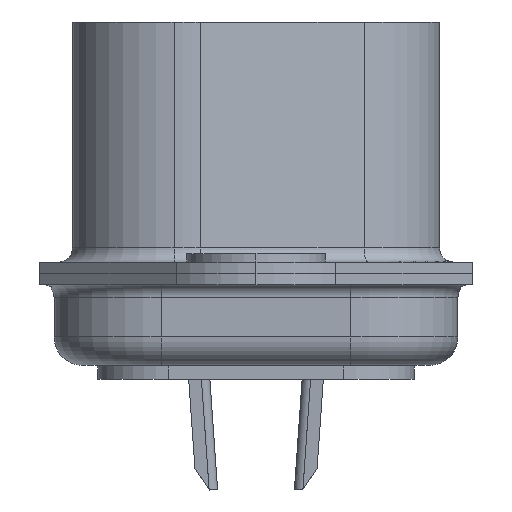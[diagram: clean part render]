
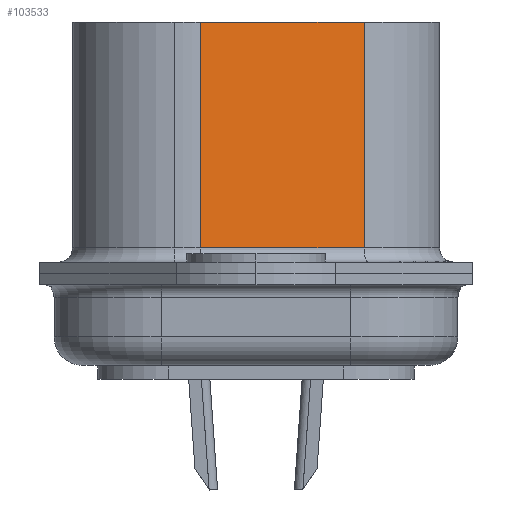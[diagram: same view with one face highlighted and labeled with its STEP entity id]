
A CAD part, left-side view. The second image highlights one B-rep face of the part: STEP entity #103533.
In plain terms, the highlighted planar face has unit normal (-0.966, -0.259, 0).
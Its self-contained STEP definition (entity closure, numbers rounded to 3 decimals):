
#7807 = ORIENTED_EDGE ( 'NONE', *, *, #25200, .T. ) ;
#22062 = PLANE ( 'NONE',  #29212 ) ;
#25200 = EDGE_CURVE ( 'NONE', #120556, #112780, #77005, .T. ) ;
#25909 = ORIENTED_EDGE ( 'NONE', *, *, #55058, .F. ) ;
#28654 = VERTEX_POINT ( 'NONE', #49153 ) ;
#29212 = AXIS2_PLACEMENT_3D ( 'NONE', #124623, #137480, #98168 ) ;
#34080 = FACE_OUTER_BOUND ( 'NONE', #68126, .T. ) ;
#49153 = CARTESIAN_POINT ( 'NONE',  ( 4.913, 1.968, 9.3 ) ) ;
#54812 = VECTOR ( 'NONE', #115452, 1000. ) ;
#55058 = EDGE_CURVE ( 'NONE', #124278, #112780, #146636, .T. ) ;
#64194 = CARTESIAN_POINT ( 'NONE',  ( 6.467, -3.832, 1.3 ) ) ;
#68126 = EDGE_LOOP ( 'NONE', ( #112509, #7807, #25909, #105767 ) ) ;
#77005 = LINE ( 'NONE', #64194, #54812 ) ;
#78291 = DIRECTION ( 'NONE',  ( 0.259, -0.966, 0. ) ) ;
#98168 = DIRECTION ( 'NONE',  ( -0.259, 0.966, 0. ) ) ;
#99212 = EDGE_CURVE ( 'NONE', #28654, #124278, #154374, .T. ) ;
#100469 = CARTESIAN_POINT ( 'NONE',  ( 4.913, 1.968, 9.3 ) ) ;
#103533 = ADVANCED_FACE ( 'NONE', ( #34080 ), #22062, .F. ) ;
#104857 = VECTOR ( 'NONE', #78291, 1000. ) ;
#105059 = CARTESIAN_POINT ( 'NONE',  ( 6.467, -3.832, 1.3 ) ) ;
#105767 = ORIENTED_EDGE ( 'NONE', *, *, #99212, .F. ) ;
#107314 = CARTESIAN_POINT ( 'NONE',  ( 6.467, -3.832, 9.3 ) ) ;
#112509 = ORIENTED_EDGE ( 'NONE', *, *, #162389, .T. ) ;
#112780 = VERTEX_POINT ( 'NONE', #105059 ) ;
#115452 = DIRECTION ( 'NONE',  ( 0.259, -0.966, 0. ) ) ;
#120556 = VERTEX_POINT ( 'NONE', #162707 ) ;
#124278 = VERTEX_POINT ( 'NONE', #157317 ) ;
#124623 = CARTESIAN_POINT ( 'NONE',  ( 6.467, -3.832, 9.3 ) ) ;
#133812 = DIRECTION ( 'NONE',  ( 0., 0., -1. ) ) ;
#137480 = DIRECTION ( 'NONE',  ( 0.966, 0.259, 0. ) ) ;
#138938 = DIRECTION ( 'NONE',  ( 0., 0., -1. ) ) ;
#146636 = LINE ( 'NONE', #107314, #156252 ) ;
#152589 = LINE ( 'NONE', #100469, #152850 ) ;
#152850 = VECTOR ( 'NONE', #138938, 1000. ) ;
#154374 = LINE ( 'NONE', #168840, #104857 ) ;
#156252 = VECTOR ( 'NONE', #133812, 1000. ) ;
#157317 = CARTESIAN_POINT ( 'NONE',  ( 6.467, -3.832, 9.3 ) ) ;
#162389 = EDGE_CURVE ( 'NONE', #28654, #120556, #152589, .T. ) ;
#162707 = CARTESIAN_POINT ( 'NONE',  ( 4.913, 1.968, 1.3 ) ) ;
#168840 = CARTESIAN_POINT ( 'NONE',  ( 6.467, -3.832, 9.3 ) ) ;
